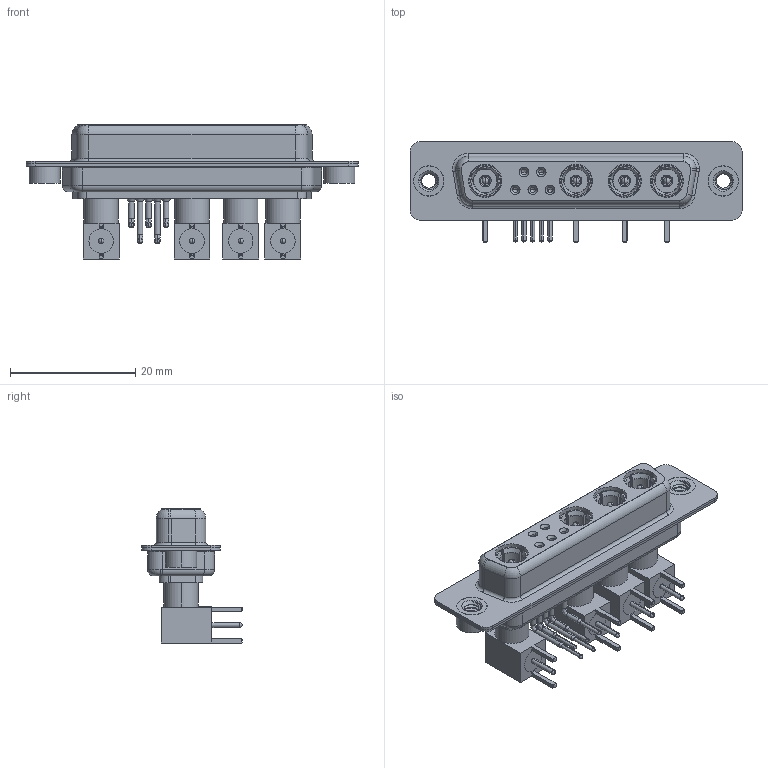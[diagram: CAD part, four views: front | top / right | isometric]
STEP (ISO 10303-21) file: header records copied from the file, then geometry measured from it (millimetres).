
FILE_DESCRIPTION (( 'STEP AP203' ), '1' );
FILE_NAME ('630-9W4-640-7T2.STEP', '2022-06-01T09:45:13', ( '' ), ( '' ), 'SwSTEP 2.0', 'SolidWorks 2020', '' );
FILE_SCHEMA (( 'CONFIG_CONTROL_DESIGN' ));
Length unit declared in the file: millimetre
Products named in the file (17): 630-9W4-640-7T2; Pin_RA; Locking Collar; 630Combo Contact Row 2; 630Combo Shell Rear_25 Contacts; 630Combo Shell Front_25 Contacts; Co-Ax Plug Assy_RA; 630Combo Housing_9W4; RA Back Shell; 630Combo Threaded Rivet_2; Insulator RA Pin; 630Combo Contact Row 1; Co-Ax Plug_RA PC Tail; Insulator Pin_Straight PC Tail
Assembly tree (38 placements, depth 3):
  630-9W4-640-7T2
    630Combo Housing_9W4
    630Combo Shell Front_25 Contacts
    630Combo Shell Rear_25 Contacts
    630Combo Threaded Rivet_2  x2
    Co-Ax Plug Assy_RA
      Co-Ax Plug_RA PC Tail
      Insulator Pin_Straight PC Tail
      Pin_RA
      Locking Collar
      RA Back Shell
      Insulator RA Pin
    Co-Ax Plug Assy_RA
      Co-Ax Plug_RA PC Tail
      Insulator Pin_Straight PC Tail
      Pin_RA
      Locking Collar
      RA Back Shell
      Insulator RA Pin
    Co-Ax Plug Assy_RA
      Co-Ax Plug_RA PC Tail
      Insulator Pin_Straight PC Tail
      Pin_RA
      Locking Collar
      RA Back Shell
      Insulator RA Pin
    Co-Ax Plug Assy_RA
      Co-Ax Plug_RA PC Tail
      Insulator Pin_Straight PC Tail
      Pin_RA
      Locking Collar
      RA Back Shell
      Insulator RA Pin
    630Combo Contact Row 1  x2
    630Combo Contact Row 2  x3
Bounding box: 53.05 x 16 x 21.41 mm (x, y, z)
Volume: 4687 mm3; surface area: 11331.6 mm2
Topology: 34 solids, 34 shells, 1216 faces, 2964 edges, 1856 vertices
Faces by surface type: cylinder 512, plane 410, cone 167, torus 81, bspline 30, sphere 16
Entity records: 21176 total; most frequent: CARTESIAN_POINT 4934, DIRECTION 3146, ORIENTED_EDGE 2750, EDGE_CURVE 1375, AXIS2_PLACEMENT_3D 1283, VERTEX_POINT 872, CIRCLE 676, EDGE_LOOP 661
